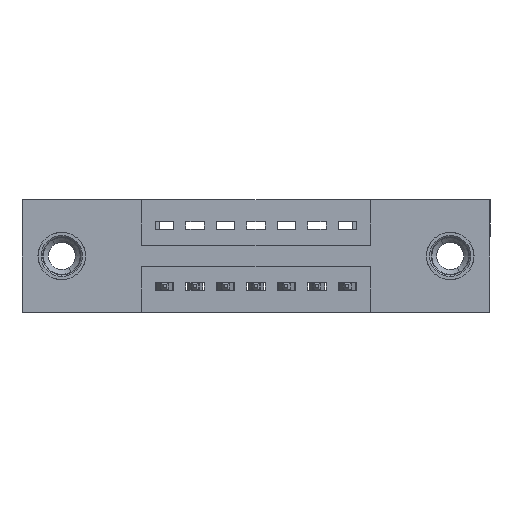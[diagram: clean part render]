
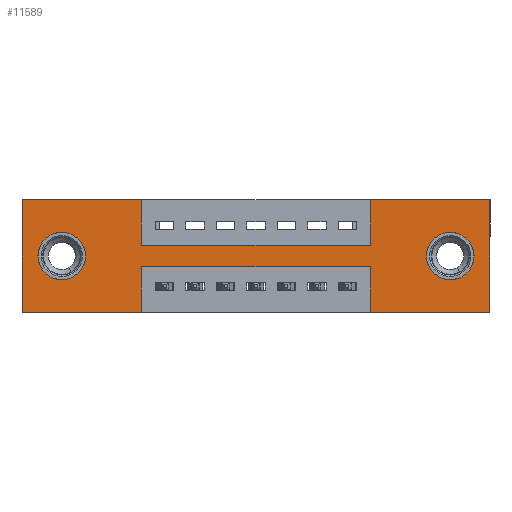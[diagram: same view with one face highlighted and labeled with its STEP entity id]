
A CAD part, front view. The second image highlights one B-rep face of the part: STEP entity #11589.
In plain terms, the highlighted planar face has unit normal (0, -1, 0).
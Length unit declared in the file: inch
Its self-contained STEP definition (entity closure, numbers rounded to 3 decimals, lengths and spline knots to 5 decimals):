
#180 = DIRECTION ( 'NONE',  ( 0., 0., -1. ) ) ;
#330 = DIRECTION ( 'NONE',  ( 0., 0., 1. ) ) ;
#381 = FACE_BOUND ( 'NONE', #7787, .T. ) ;
#434 = VECTOR ( 'NONE', #5338, 39.37008 ) ;
#572 = ORIENTED_EDGE ( 'NONE', *, *, #8316, .F. ) ;
#616 = CIRCLE ( 'NONE', #4991, 0.078 ) ;
#684 = DIRECTION ( 'NONE',  ( 0., 0., -1. ) ) ;
#809 = EDGE_CURVE ( 'NONE', #6306, #8848, #2117, .T. ) ;
#838 = CARTESIAN_POINT ( 'NONE',  ( 0.3925, 0., -0.15 ) ) ;
#906 = DIRECTION ( 'NONE',  ( 0., 0., 1. ) ) ;
#939 = LINE ( 'NONE', #5893, #10594 ) ;
#1044 = ORIENTED_EDGE ( 'NONE', *, *, #809, .F. ) ;
#1119 = CARTESIAN_POINT ( 'NONE',  ( 1.1425, 0., -0.22 ) ) ;
#1414 = CARTESIAN_POINT ( 'NONE',  ( 0., 0., 0. ) ) ;
#1550 = EDGE_CURVE ( 'NONE', #8133, #5523, #5325, .T. ) ;
#1572 = EDGE_CURVE ( 'NONE', #5523, #8133, #4003, .T. ) ;
#1600 = VERTEX_POINT ( 'NONE', #4428 ) ;
#1692 = CARTESIAN_POINT ( 'NONE',  ( 0.13, 0., -0.185 ) ) ;
#1882 = ORIENTED_EDGE ( 'NONE', *, *, #2818, .F. ) ;
#2117 = LINE ( 'NONE', #3315, #8694 ) ;
#2146 = EDGE_CURVE ( 'NONE', #5974, #6306, #8841, .T. ) ;
#2305 = VERTEX_POINT ( 'NONE', #3707 ) ;
#2315 = ORIENTED_EDGE ( 'NONE', *, *, #6305, .F. ) ;
#2365 = ORIENTED_EDGE ( 'NONE', *, *, #7334, .F. ) ;
#2552 = CARTESIAN_POINT ( 'NONE',  ( 0.13, 0., -0.263 ) ) ;
#2723 = VECTOR ( 'NONE', #180, 39.37008 ) ;
#2738 = CARTESIAN_POINT ( 'NONE',  ( 1.1425, 0., -0.37 ) ) ;
#2758 = VECTOR ( 'NONE', #330, 39.37008 ) ;
#2818 = EDGE_CURVE ( 'NONE', #6668, #2305, #939, .T. ) ;
#2919 = ORIENTED_EDGE ( 'NONE', *, *, #3095, .F. ) ;
#3072 = CARTESIAN_POINT ( 'NONE',  ( 1.405, 0., -0.263 ) ) ;
#3095 = EDGE_CURVE ( 'NONE', #9079, #6668, #8107, .T. ) ;
#3101 = PLANE ( 'NONE',  #5104 ) ;
#3111 = CARTESIAN_POINT ( 'NONE',  ( 0.3925, 0., -0.15 ) ) ;
#3142 = DIRECTION ( 'NONE',  ( 0., -1., 0. ) ) ;
#3312 = ORIENTED_EDGE ( 'NONE', *, *, #8405, .T. ) ;
#3315 = CARTESIAN_POINT ( 'NONE',  ( 0., 0., -0.37 ) ) ;
#3330 = CIRCLE ( 'NONE', #7691, 0.078 ) ;
#3413 = CARTESIAN_POINT ( 'NONE',  ( 1.405, 0., -0.185 ) ) ;
#3690 = CARTESIAN_POINT ( 'NONE',  ( 0., 0., -0.37 ) ) ;
#3707 = CARTESIAN_POINT ( 'NONE',  ( 0.3925, 0., 0. ) ) ;
#3750 = VECTOR ( 'NONE', #4616, 39.37008 ) ;
#3832 = VERTEX_POINT ( 'NONE', #8120 ) ;
#4003 = CIRCLE ( 'NONE', #8463, 0.078 ) ;
#4074 = CARTESIAN_POINT ( 'NONE',  ( 1.535, 0., 0. ) ) ;
#4089 = CARTESIAN_POINT ( 'NONE',  ( 0., 0., 0. ) ) ;
#4263 = VECTOR ( 'NONE', #5383, 39.37008 ) ;
#4271 = DIRECTION ( 'NONE',  ( 0., 0., -1. ) ) ;
#4292 = VECTOR ( 'NONE', #906, 39.37008 ) ;
#4361 = DIRECTION ( 'NONE',  ( -1., 0., 0. ) ) ;
#4362 = EDGE_CURVE ( 'NONE', #7845, #5285, #9704, .T. ) ;
#4428 = CARTESIAN_POINT ( 'NONE',  ( 0.3925, 0., -0.37 ) ) ;
#4479 = ORIENTED_EDGE ( 'NONE', *, *, #6758, .F. ) ;
#4616 = DIRECTION ( 'NONE',  ( 0., 0., 1. ) ) ;
#4744 = CARTESIAN_POINT ( 'NONE',  ( 0.3925, 0., 0. ) ) ;
#4943 = VECTOR ( 'NONE', #8492, 39.37008 ) ;
#4987 = DIRECTION ( 'NONE',  ( 1., 0., 0. ) ) ;
#4991 = AXIS2_PLACEMENT_3D ( 'NONE', #9977, #6238, #8143 ) ;
#5069 = ORIENTED_EDGE ( 'NONE', *, *, #10806, .T. ) ;
#5104 = AXIS2_PLACEMENT_3D ( 'NONE', #6844, #3142, #6759 ) ;
#5205 = LINE ( 'NONE', #10442, #2723 ) ;
#5207 = CARTESIAN_POINT ( 'NONE',  ( 1.1425, 0., -0.37 ) ) ;
#5238 = LINE ( 'NONE', #4744, #4943 ) ;
#5285 = VERTEX_POINT ( 'NONE', #10047 ) ;
#5314 = DIRECTION ( 'NONE',  ( 0., 1., 0. ) ) ;
#5325 = CIRCLE ( 'NONE', #10926, 0.078 ) ;
#5338 = DIRECTION ( 'NONE',  ( -1., 0., 0. ) ) ;
#5363 = VERTEX_POINT ( 'NONE', #2552 ) ;
#5381 = VECTOR ( 'NONE', #6982, 39.37008 ) ;
#5383 = DIRECTION ( 'NONE',  ( -1., 0., 0. ) ) ;
#5523 = VERTEX_POINT ( 'NONE', #10858 ) ;
#5530 = VERTEX_POINT ( 'NONE', #6207 ) ;
#5532 = LINE ( 'NONE', #8216, #434 ) ;
#5540 = ORIENTED_EDGE ( 'NONE', *, *, #1572, .T. ) ;
#5629 = VECTOR ( 'NONE', #11697, 39.37008 ) ;
#5893 = CARTESIAN_POINT ( 'NONE',  ( 0., 0., 0. ) ) ;
#5974 = VERTEX_POINT ( 'NONE', #4074 ) ;
#6081 = CARTESIAN_POINT ( 'NONE',  ( 0.3925, 0., -0.22 ) ) ;
#6134 = EDGE_CURVE ( 'NONE', #2305, #7845, #5238, .T. ) ;
#6207 = CARTESIAN_POINT ( 'NONE',  ( 0.3925, 0., -0.22 ) ) ;
#6238 = DIRECTION ( 'NONE',  ( 0., 1., 0. ) ) ;
#6305 = EDGE_CURVE ( 'NONE', #5285, #11694, #6698, .T. ) ;
#6306 = VERTEX_POINT ( 'NONE', #10635 ) ;
#6339 = DIRECTION ( 'NONE',  ( 0., 1., 0. ) ) ;
#6658 = LINE ( 'NONE', #2738, #3750 ) ;
#6668 = VERTEX_POINT ( 'NONE', #1414 ) ;
#6698 = LINE ( 'NONE', #8725, #2758 ) ;
#6723 = ORIENTED_EDGE ( 'NONE', *, *, #6134, .F. ) ;
#6758 = EDGE_CURVE ( 'NONE', #1600, #9079, #5532, .T. ) ;
#6759 = DIRECTION ( 'NONE',  ( 0., 0., -1. ) ) ;
#6787 = FACE_OUTER_BOUND ( 'NONE', #8617, .T. ) ;
#6844 = CARTESIAN_POINT ( 'NONE',  ( 0., 0., -0.37 ) ) ;
#6966 = ORIENTED_EDGE ( 'NONE', *, *, #9995, .F. ) ;
#6982 = DIRECTION ( 'NONE',  ( 1., 0., 0. ) ) ;
#7183 = ORIENTED_EDGE ( 'NONE', *, *, #2146, .F. ) ;
#7328 = DIRECTION ( 'NONE',  ( 0., 0., 1. ) ) ;
#7334 = EDGE_CURVE ( 'NONE', #8848, #9896, #6658, .T. ) ;
#7684 = FACE_BOUND ( 'NONE', #9326, .T. ) ;
#7691 = AXIS2_PLACEMENT_3D ( 'NONE', #1692, #6339, #7328 ) ;
#7787 = EDGE_LOOP ( 'NONE', ( #5069, #3312 ) ) ;
#7845 = VERTEX_POINT ( 'NONE', #838 ) ;
#7939 = VECTOR ( 'NONE', #4987, 39.37008 ) ;
#8107 = LINE ( 'NONE', #10309, #4292 ) ;
#8120 = CARTESIAN_POINT ( 'NONE',  ( 0.13, 0., -0.107 ) ) ;
#8133 = VERTEX_POINT ( 'NONE', #3072 ) ;
#8143 = DIRECTION ( 'NONE',  ( 0., 0., 1. ) ) ;
#8216 = CARTESIAN_POINT ( 'NONE',  ( 0., 0., -0.37 ) ) ;
#8316 = EDGE_CURVE ( 'NONE', #9896, #5530, #9388, .T. ) ;
#8405 = EDGE_CURVE ( 'NONE', #5363, #3832, #616, .T. ) ;
#8463 = AXIS2_PLACEMENT_3D ( 'NONE', #10955, #5314, #684 ) ;
#8492 = DIRECTION ( 'NONE',  ( 0., 0., -1. ) ) ;
#8617 = EDGE_LOOP ( 'NONE', ( #8851, #572, #2365, #1044, #7183, #6966, #2315, #10880, #6723, #1882, #2919, #4479 ) ) ;
#8694 = VECTOR ( 'NONE', #4361, 39.37008 ) ;
#8725 = CARTESIAN_POINT ( 'NONE',  ( 1.1425, 0., 0. ) ) ;
#8841 = LINE ( 'NONE', #11739, #5629 ) ;
#8848 = VERTEX_POINT ( 'NONE', #5207 ) ;
#8851 = ORIENTED_EDGE ( 'NONE', *, *, #11044, .F. ) ;
#9079 = VERTEX_POINT ( 'NONE', #3690 ) ;
#9326 = EDGE_LOOP ( 'NONE', ( #5540, #11064 ) ) ;
#9388 = LINE ( 'NONE', #6081, #4263 ) ;
#9608 = DIRECTION ( 'NONE',  ( 1., 0., 0. ) ) ;
#9704 = LINE ( 'NONE', #3111, #7939 ) ;
#9896 = VERTEX_POINT ( 'NONE', #1119 ) ;
#9956 = DIRECTION ( 'NONE',  ( 0., 1., 0. ) ) ;
#9977 = CARTESIAN_POINT ( 'NONE',  ( 0.13, 0., -0.185 ) ) ;
#9995 = EDGE_CURVE ( 'NONE', #11694, #5974, #11275, .T. ) ;
#10047 = CARTESIAN_POINT ( 'NONE',  ( 1.1425, 0., -0.15 ) ) ;
#10309 = CARTESIAN_POINT ( 'NONE',  ( 0., 0., 0. ) ) ;
#10442 = CARTESIAN_POINT ( 'NONE',  ( 0.3925, 0., -0.37 ) ) ;
#10594 = VECTOR ( 'NONE', #9608, 39.37008 ) ;
#10635 = CARTESIAN_POINT ( 'NONE',  ( 1.535, 0., -0.37 ) ) ;
#10806 = EDGE_CURVE ( 'NONE', #3832, #5363, #3330, .T. ) ;
#10858 = CARTESIAN_POINT ( 'NONE',  ( 1.405, 0., -0.107 ) ) ;
#10880 = ORIENTED_EDGE ( 'NONE', *, *, #4362, .F. ) ;
#10926 = AXIS2_PLACEMENT_3D ( 'NONE', #3413, #9956, #4271 ) ;
#10955 = CARTESIAN_POINT ( 'NONE',  ( 1.405, 0., -0.185 ) ) ;
#11044 = EDGE_CURVE ( 'NONE', #5530, #1600, #5205, .T. ) ;
#11064 = ORIENTED_EDGE ( 'NONE', *, *, #1550, .T. ) ;
#11275 = LINE ( 'NONE', #4089, #5381 ) ;
#11589 = ADVANCED_FACE ( 'NONE', ( #7684, #381, #6787 ), #3101, .T. ) ;
#11636 = CARTESIAN_POINT ( 'NONE',  ( 1.1425, 0., 0. ) ) ;
#11694 = VERTEX_POINT ( 'NONE', #11636 ) ;
#11697 = DIRECTION ( 'NONE',  ( 0., 0., -1. ) ) ;
#11739 = CARTESIAN_POINT ( 'NONE',  ( 1.535, 0., 0. ) ) ;
